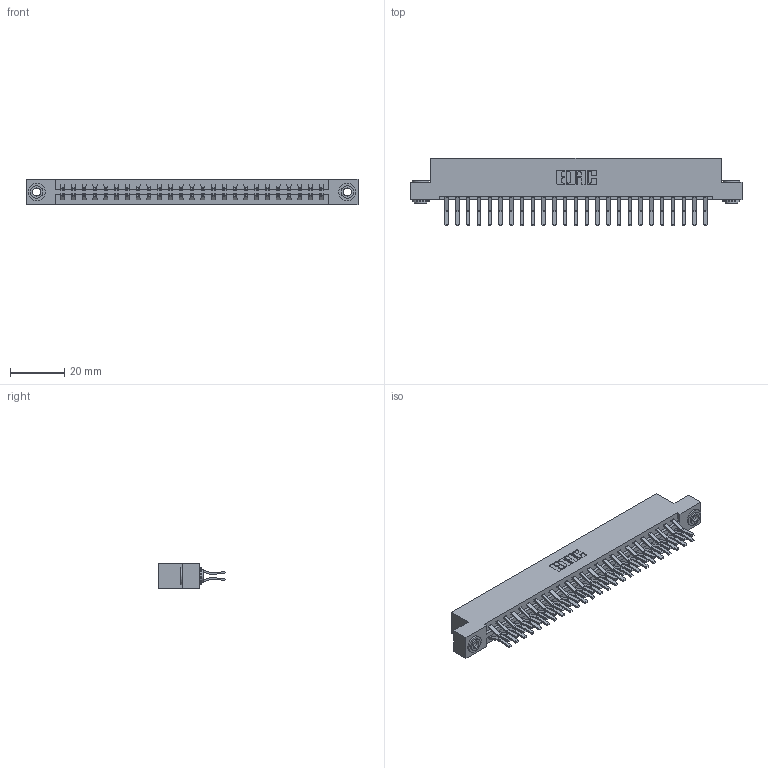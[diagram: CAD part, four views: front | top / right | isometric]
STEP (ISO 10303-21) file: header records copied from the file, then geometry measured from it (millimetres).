
FILE_DESCRIPTION (( 'STEP AP203' ), '1' );
FILE_NAME ('337-050-560-203.STEP', '2018-08-09T21:53:18', ( '' ), ( '' ), 'SwSTEP 2.0', 'SolidWorks 2016', '' );
FILE_SCHEMA (( 'CONFIG_CONTROL_DESIGN' ));
Length unit declared in the file: inch
Products named in the file (4): 345-250-002_345-250-002-102; 337-050-560-203; 337 Part_Flush Mounting Lugs - 0.156 Dia-TH; 345-292-001_560 Tail
Assembly tree (53 placements, depth 2):
  337-050-560-203
    337 Part_Flush Mounting Lugs - 0.156 Dia-TH
    345-292-001_560 Tail  x50
    345-250-002_345-250-002-102  x2
Bounding box: 122.07 x 24.78 x 9.4 mm (x, y, z)
Volume: 12985.8 mm3; surface area: 15688.3 mm2
Topology: 53 solids, 53 shells, 2952 faces, 8737 edges, 5754 vertices
Faces by surface type: plane 1980, cylinder 964, cone 8
Entity records: 22320 total; most frequent: CARTESIAN_POINT 3749, ORIENTED_EDGE 3678, DIRECTION 3257, EDGE_CURVE 1839, VECTOR 1683, LINE 1683, VERTEX_POINT 1222, AXIS2_PLACEMENT_3D 787
